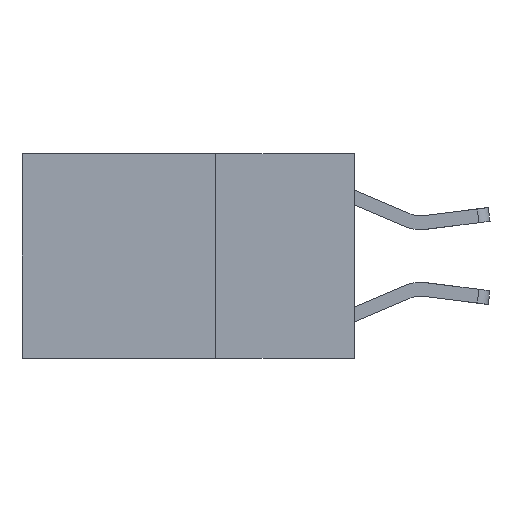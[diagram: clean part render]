
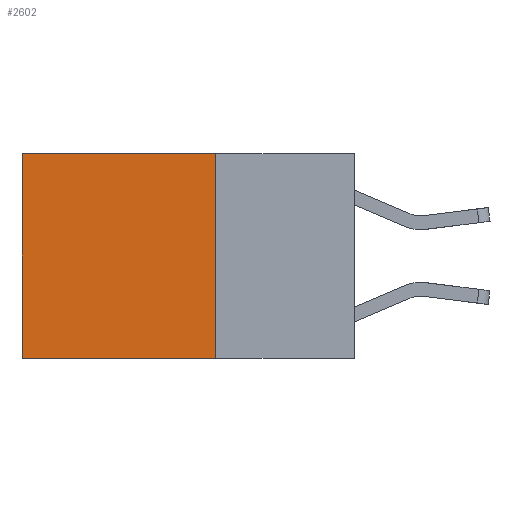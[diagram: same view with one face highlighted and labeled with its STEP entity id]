
A CAD part, left-side view. The second image highlights one B-rep face of the part: STEP entity #2602.
In plain terms, the highlighted planar face has unit normal (-1, 0, 0).
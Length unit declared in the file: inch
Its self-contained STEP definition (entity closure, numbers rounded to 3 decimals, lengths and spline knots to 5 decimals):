
#645 = DIRECTION ( 'NONE',  ( 0., 1., 0. ) ) ;
#869 = LINE ( 'NONE', #7194, #2215 ) ;
#1115 = ORIENTED_EDGE ( 'NONE', *, *, #5583, .T. ) ;
#1183 = PLANE ( 'NONE',  #1491 ) ;
#1263 = CARTESIAN_POINT ( 'NONE',  ( 0.2625, 0.6, -0.37 ) ) ;
#1281 = DIRECTION ( 'NONE',  ( 1., 0., 0. ) ) ;
#1491 = AXIS2_PLACEMENT_3D ( 'NONE', #2632, #1281, #4579 ) ;
#1751 = LINE ( 'NONE', #5221, #5564 ) ;
#2215 = VECTOR ( 'NONE', #3763, 39.37008 ) ;
#2554 = CARTESIAN_POINT ( 'NONE',  ( 0.2625, 0.25, -0.37 ) ) ;
#2602 = ADVANCED_FACE ( 'NONE', ( #6663 ), #1183, .F. ) ;
#2632 = CARTESIAN_POINT ( 'NONE',  ( 0.2625, 0.25, 0. ) ) ;
#3298 = CARTESIAN_POINT ( 'NONE',  ( 0.2625, 0.25, 0. ) ) ;
#3404 = ORIENTED_EDGE ( 'NONE', *, *, #8856, .T. ) ;
#3606 = EDGE_CURVE ( 'NONE', #3707, #6809, #6219, .T. ) ;
#3707 = VERTEX_POINT ( 'NONE', #3298 ) ;
#3718 = VECTOR ( 'NONE', #645, 39.37008 ) ;
#3763 = DIRECTION ( 'NONE',  ( 0., 1., 0. ) ) ;
#4111 = VERTEX_POINT ( 'NONE', #1263 ) ;
#4447 = ORIENTED_EDGE ( 'NONE', *, *, #3606, .F. ) ;
#4579 = DIRECTION ( 'NONE',  ( 0., 0., -1. ) ) ;
#4768 = DIRECTION ( 'NONE',  ( 0., 0., -1. ) ) ;
#4804 = CARTESIAN_POINT ( 'NONE',  ( 0.2625, 0.6, 0. ) ) ;
#4833 = ORIENTED_EDGE ( 'NONE', *, *, #8160, .F. ) ;
#5181 = DIRECTION ( 'NONE',  ( 0., 0., -1. ) ) ;
#5221 = CARTESIAN_POINT ( 'NONE',  ( 0.2625, 0.6, 0. ) ) ;
#5307 = LINE ( 'NONE', #2554, #3718 ) ;
#5492 = CARTESIAN_POINT ( 'NONE',  ( 0.2625, 0.25, 0. ) ) ;
#5564 = VECTOR ( 'NONE', #5181, 39.37008 ) ;
#5583 = EDGE_CURVE ( 'NONE', #6184, #4111, #1751, .T. ) ;
#6184 = VERTEX_POINT ( 'NONE', #4804 ) ;
#6219 = LINE ( 'NONE', #5492, #6403 ) ;
#6403 = VECTOR ( 'NONE', #4768, 39.37008 ) ;
#6663 = FACE_OUTER_BOUND ( 'NONE', #7897, .T. ) ;
#6809 = VERTEX_POINT ( 'NONE', #7670 ) ;
#7194 = CARTESIAN_POINT ( 'NONE',  ( 0.2625, 0.25, 0. ) ) ;
#7670 = CARTESIAN_POINT ( 'NONE',  ( 0.2625, 0.25, -0.37 ) ) ;
#7897 = EDGE_LOOP ( 'NONE', ( #1115, #4833, #4447, #3404 ) ) ;
#8160 = EDGE_CURVE ( 'NONE', #6809, #4111, #5307, .T. ) ;
#8856 = EDGE_CURVE ( 'NONE', #3707, #6184, #869, .T. ) ;
